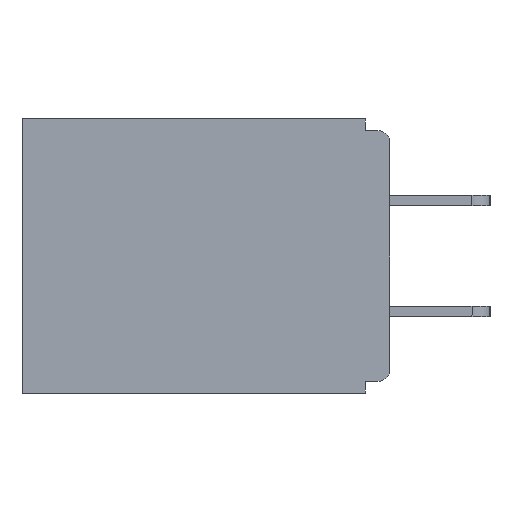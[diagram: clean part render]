
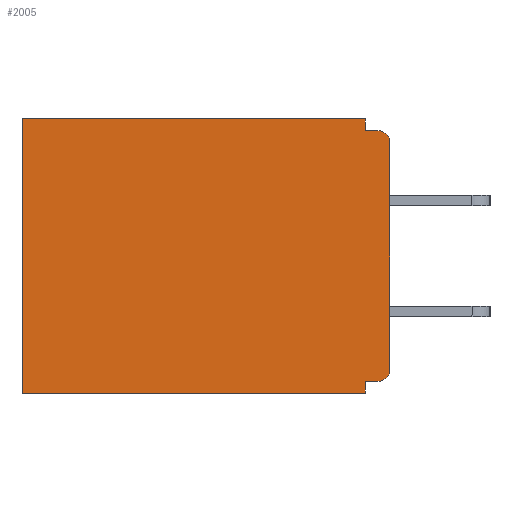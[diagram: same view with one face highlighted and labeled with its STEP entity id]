
A CAD part, left-side view. The second image highlights one B-rep face of the part: STEP entity #2005.
In plain terms, the highlighted planar face has unit normal (-1, 0, 0).
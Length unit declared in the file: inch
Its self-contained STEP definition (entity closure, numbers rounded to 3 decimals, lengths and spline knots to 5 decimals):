
#109 = DIRECTION ( 'NONE',  ( 0., 1., 0. ) ) ;
#223 = VERTEX_POINT ( 'NONE', #1104 ) ;
#274 = CARTESIAN_POINT ( 'NONE',  ( 0.298, 0.46, 0. ) ) ;
#418 = VERTEX_POINT ( 'NONE', #4023 ) ;
#774 = DIRECTION ( 'NONE',  ( 0., 0., -1. ) ) ;
#829 = CARTESIAN_POINT ( 'NONE',  ( 0.298, 0., -0.328 ) ) ;
#904 = VERTEX_POINT ( 'NONE', #9737 ) ;
#1104 = CARTESIAN_POINT ( 'NONE',  ( 0.298, 0.015, -0.015 ) ) ;
#1192 = AXIS2_PLACEMENT_3D ( 'NONE', #8087, #4036, #5693 ) ;
#1285 = CARTESIAN_POINT ( 'NONE',  ( 0.298, 0.031, -0.343 ) ) ;
#1289 = VECTOR ( 'NONE', #9878, 39.37008 ) ;
#1588 = EDGE_CURVE ( 'NONE', #4093, #223, #8608, .T. ) ;
#1802 = LINE ( 'NONE', #4337, #1289 ) ;
#1836 = ORIENTED_EDGE ( 'NONE', *, *, #1588, .F. ) ;
#2005 = ADVANCED_FACE ( 'NONE', ( #2376 ), #4010, .F. ) ;
#2335 = EDGE_CURVE ( 'NONE', #5838, #4782, #6546, .T. ) ;
#2376 = FACE_OUTER_BOUND ( 'NONE', #3085, .T. ) ;
#2386 = EDGE_CURVE ( 'NONE', #10419, #10214, #10449, .T. ) ;
#2457 = CIRCLE ( 'NONE', #4357, 0.015 ) ;
#2893 = CARTESIAN_POINT ( 'NONE',  ( 0.298, 0.031, -0.328 ) ) ;
#2927 = ORIENTED_EDGE ( 'NONE', *, *, #4640, .T. ) ;
#2983 = EDGE_CURVE ( 'NONE', #904, #223, #2457, .T. ) ;
#3077 = LINE ( 'NONE', #274, #3974 ) ;
#3085 = EDGE_LOOP ( 'NONE', ( #4712, #1836, #10037, #8012, #2927, #8429, #6259, #7142, #9784, #7137 ) ) ;
#3187 = VECTOR ( 'NONE', #4687, 39.37008 ) ;
#3468 = DIRECTION ( 'NONE',  ( 0., 0., -1. ) ) ;
#3600 = CARTESIAN_POINT ( 'NONE',  ( 0.298, 0., -0.313 ) ) ;
#3677 = DIRECTION ( 'NONE',  ( 0., -1., 0. ) ) ;
#3817 = VERTEX_POINT ( 'NONE', #8387 ) ;
#3974 = VECTOR ( 'NONE', #3468, 39.37008 ) ;
#4010 = PLANE ( 'NONE',  #1192 ) ;
#4016 = DIRECTION ( 'NONE',  ( -1., 0., 0. ) ) ;
#4023 = CARTESIAN_POINT ( 'NONE',  ( 0.298, 0.031, 0. ) ) ;
#4036 = DIRECTION ( 'NONE',  ( 1., 0., 0. ) ) ;
#4093 = VERTEX_POINT ( 'NONE', #8105 ) ;
#4127 = DIRECTION ( 'NONE',  ( 0., 1., 0. ) ) ;
#4337 = CARTESIAN_POINT ( 'NONE',  ( 0.298, 0., 0. ) ) ;
#4357 = AXIS2_PLACEMENT_3D ( 'NONE', #10333, #8762, #6245 ) ;
#4434 = VECTOR ( 'NONE', #5818, 39.37008 ) ;
#4442 = EDGE_CURVE ( 'NONE', #5838, #5176, #7774, .T. ) ;
#4625 = CARTESIAN_POINT ( 'NONE',  ( 0.298, 0.031, -0.343 ) ) ;
#4640 = EDGE_CURVE ( 'NONE', #3817, #10214, #3077, .T. ) ;
#4653 = EDGE_CURVE ( 'NONE', #418, #3817, #1802, .T. ) ;
#4687 = DIRECTION ( 'NONE',  ( 0., 0., -1. ) ) ;
#4709 = VECTOR ( 'NONE', #4932, 39.37008 ) ;
#4712 = ORIENTED_EDGE ( 'NONE', *, *, #2983, .T. ) ;
#4782 = VERTEX_POINT ( 'NONE', #2893 ) ;
#4932 = DIRECTION ( 'NONE',  ( 0., 0., -1. ) ) ;
#4995 = EDGE_CURVE ( 'NONE', #418, #4093, #6879, .T. ) ;
#5176 = VERTEX_POINT ( 'NONE', #3600 ) ;
#5214 = EDGE_CURVE ( 'NONE', #4782, #10419, #7372, .T. ) ;
#5546 = EDGE_CURVE ( 'NONE', #904, #5176, #9660, .T. ) ;
#5693 = DIRECTION ( 'NONE',  ( 0., 0., -1. ) ) ;
#5717 = CARTESIAN_POINT ( 'NONE',  ( 0.298, 0., -0.343 ) ) ;
#5818 = DIRECTION ( 'NONE',  ( 0., 0., -1. ) ) ;
#5838 = VERTEX_POINT ( 'NONE', #8292 ) ;
#6144 = CARTESIAN_POINT ( 'NONE',  ( 0.298, 0.46, -0.343 ) ) ;
#6245 = DIRECTION ( 'NONE',  ( 0., 0., -1. ) ) ;
#6259 = ORIENTED_EDGE ( 'NONE', *, *, #5214, .F. ) ;
#6317 = CARTESIAN_POINT ( 'NONE',  ( 0.298, 0.015, -0.313 ) ) ;
#6546 = LINE ( 'NONE', #829, #10021 ) ;
#6605 = CARTESIAN_POINT ( 'NONE',  ( 0.298, 0., 0. ) ) ;
#6879 = LINE ( 'NONE', #10046, #4709 ) ;
#7137 = ORIENTED_EDGE ( 'NONE', *, *, #5546, .F. ) ;
#7142 = ORIENTED_EDGE ( 'NONE', *, *, #2335, .F. ) ;
#7208 = VECTOR ( 'NONE', #3677, 39.37008 ) ;
#7300 = VECTOR ( 'NONE', #109, 39.37008 ) ;
#7372 = LINE ( 'NONE', #4625, #3187 ) ;
#7478 = CARTESIAN_POINT ( 'NONE',  ( 0.298, 0., -0.015 ) ) ;
#7703 = AXIS2_PLACEMENT_3D ( 'NONE', #6317, #4016, #774 ) ;
#7774 = CIRCLE ( 'NONE', #7703, 0.015 ) ;
#8012 = ORIENTED_EDGE ( 'NONE', *, *, #4653, .T. ) ;
#8087 = CARTESIAN_POINT ( 'NONE',  ( 0.298, 0., 0. ) ) ;
#8105 = CARTESIAN_POINT ( 'NONE',  ( 0.298, 0.031, -0.015 ) ) ;
#8292 = CARTESIAN_POINT ( 'NONE',  ( 0.298, 0.015, -0.328 ) ) ;
#8387 = CARTESIAN_POINT ( 'NONE',  ( 0.298, 0.46, 0. ) ) ;
#8429 = ORIENTED_EDGE ( 'NONE', *, *, #2386, .F. ) ;
#8608 = LINE ( 'NONE', #7478, #7208 ) ;
#8762 = DIRECTION ( 'NONE',  ( -1., 0., 0. ) ) ;
#9660 = LINE ( 'NONE', #6605, #4434 ) ;
#9737 = CARTESIAN_POINT ( 'NONE',  ( 0.298, 0., -0.03 ) ) ;
#9784 = ORIENTED_EDGE ( 'NONE', *, *, #4442, .T. ) ;
#9878 = DIRECTION ( 'NONE',  ( 0., 1., 0. ) ) ;
#10021 = VECTOR ( 'NONE', #4127, 39.37008 ) ;
#10037 = ORIENTED_EDGE ( 'NONE', *, *, #4995, .F. ) ;
#10046 = CARTESIAN_POINT ( 'NONE',  ( 0.298, 0.031, -0.343 ) ) ;
#10214 = VERTEX_POINT ( 'NONE', #6144 ) ;
#10333 = CARTESIAN_POINT ( 'NONE',  ( 0.298, 0.015, -0.03 ) ) ;
#10419 = VERTEX_POINT ( 'NONE', #1285 ) ;
#10449 = LINE ( 'NONE', #5717, #7300 ) ;
